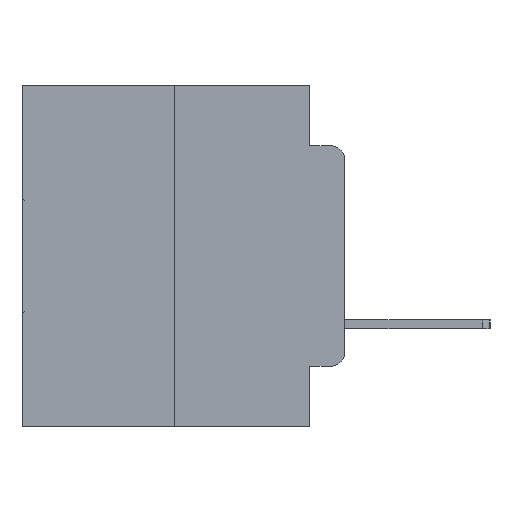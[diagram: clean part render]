
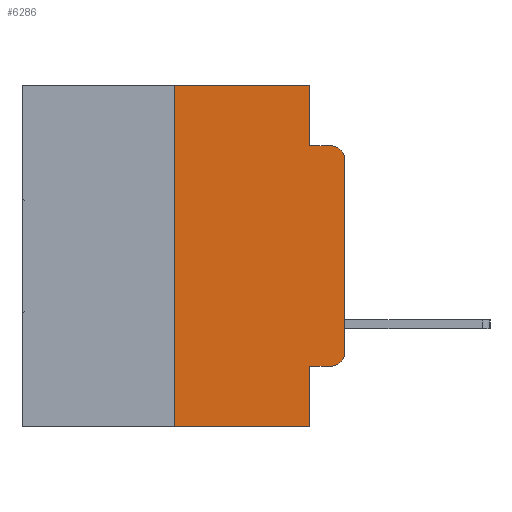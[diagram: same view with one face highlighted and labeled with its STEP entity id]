
A CAD part, left-side view. The second image highlights one B-rep face of the part: STEP entity #6286.
In plain terms, the highlighted planar face has unit normal (-1, 0, 0).
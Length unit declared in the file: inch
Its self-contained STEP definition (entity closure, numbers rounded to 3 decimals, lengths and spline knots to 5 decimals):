
#160 = CARTESIAN_POINT ( 'NONE',  ( 0., 0., -0.1085 ) ) ;
#285 = EDGE_CURVE ( 'NONE', #18609, #29116, #14256, .T. ) ;
#419 = LINE ( 'NONE', #23918, #28640 ) ;
#1270 = VERTEX_POINT ( 'NONE', #28514 ) ;
#1973 = EDGE_CURVE ( 'NONE', #26638, #18609, #24663, .T. ) ;
#2073 = LINE ( 'NONE', #5348, #7656 ) ;
#2400 = ORIENTED_EDGE ( 'NONE', *, *, #21439, .T. ) ;
#2873 = LINE ( 'NONE', #26602, #19403 ) ;
#3218 = EDGE_CURVE ( 'NONE', #14050, #19215, #4647, .T. ) ;
#3856 = CARTESIAN_POINT ( 'NONE',  ( 0., 0.02, -0.3915 ) ) ;
#4589 = AXIS2_PLACEMENT_3D ( 'NONE', #22529, #22428, #27121 ) ;
#4647 = LINE ( 'NONE', #22957, #28654 ) ;
#5004 = ORIENTED_EDGE ( 'NONE', *, *, #1973, .T. ) ;
#5060 = DIRECTION ( 'NONE',  ( 0., -1., 0. ) ) ;
#5348 = CARTESIAN_POINT ( 'NONE',  ( 0., 0.051, -0.4115 ) ) ;
#5400 = CARTESIAN_POINT ( 'NONE',  ( 0., 0., 0. ) ) ;
#5578 = VECTOR ( 'NONE', #5060, 39.37008 ) ;
#6203 = DIRECTION ( 'NONE',  ( 0., 0., -1. ) ) ;
#6286 = ADVANCED_FACE ( 'NONE', ( #17348 ), #24834, .F. ) ;
#6329 = VERTEX_POINT ( 'NONE', #27222 ) ;
#7656 = VECTOR ( 'NONE', #26346, 39.37008 ) ;
#7874 = VERTEX_POINT ( 'NONE', #24130 ) ;
#8524 = DIRECTION ( 'NONE',  ( 0., 0., -1. ) ) ;
#8939 = CARTESIAN_POINT ( 'NONE',  ( 0., 0.25, 0. ) ) ;
#8965 = EDGE_CURVE ( 'NONE', #14423, #1270, #2073, .T. ) ;
#9714 = CARTESIAN_POINT ( 'NONE',  ( 0., 0.051, 0. ) ) ;
#9726 = CARTESIAN_POINT ( 'NONE',  ( 0., 0.051, -0.0885 ) ) ;
#11994 = VERTEX_POINT ( 'NONE', #24104 ) ;
#12165 = EDGE_CURVE ( 'NONE', #14423, #11994, #23568, .T. ) ;
#12405 = CARTESIAN_POINT ( 'NONE',  ( 0., 0., -0.3915 ) ) ;
#13073 = VECTOR ( 'NONE', #24089, 39.37008 ) ;
#13245 = CARTESIAN_POINT ( 'NONE',  ( 0., 0.02, -0.1085 ) ) ;
#13515 = ORIENTED_EDGE ( 'NONE', *, *, #19920, .F. ) ;
#13523 = AXIS2_PLACEMENT_3D ( 'NONE', #3856, #20240, #6203 ) ;
#14050 = VERTEX_POINT ( 'NONE', #8939 ) ;
#14256 = CIRCLE ( 'NONE', #28641, 0.02 ) ;
#14423 = VERTEX_POINT ( 'NONE', #19727 ) ;
#14699 = DIRECTION ( 'NONE',  ( 0., 0., 1. ) ) ;
#15256 = EDGE_CURVE ( 'NONE', #7874, #14050, #419, .T. ) ;
#15309 = EDGE_LOOP ( 'NONE', ( #5004, #29695, #18971, #13515, #20412, #26522, #2400, #21862, #27959, #17120 ) ) ;
#15576 = DIRECTION ( 'NONE',  ( 0., 0., -1. ) ) ;
#16053 = DIRECTION ( 'NONE',  ( 0., -1., 0. ) ) ;
#16829 = CARTESIAN_POINT ( 'NONE',  ( 0., 0.473, -0.5 ) ) ;
#17120 = ORIENTED_EDGE ( 'NONE', *, *, #29683, .T. ) ;
#17348 = FACE_OUTER_BOUND ( 'NONE', #15309, .T. ) ;
#17412 = DIRECTION ( 'NONE',  ( 0., 0., -1. ) ) ;
#18609 = VERTEX_POINT ( 'NONE', #160 ) ;
#18971 = ORIENTED_EDGE ( 'NONE', *, *, #26090, .F. ) ;
#19198 = DIRECTION ( 'NONE',  ( 0., -1., 0. ) ) ;
#19215 = VERTEX_POINT ( 'NONE', #9714 ) ;
#19403 = VECTOR ( 'NONE', #17412, 39.37008 ) ;
#19727 = CARTESIAN_POINT ( 'NONE',  ( 0., 0.051, -0.4115 ) ) ;
#19822 = CIRCLE ( 'NONE', #13523, 0.02 ) ;
#19920 = EDGE_CURVE ( 'NONE', #19215, #6329, #2873, .T. ) ;
#20068 = CARTESIAN_POINT ( 'NONE',  ( 0., 0.02, -0.0885 ) ) ;
#20163 = CARTESIAN_POINT ( 'NONE',  ( 0., 0.051, 0. ) ) ;
#20240 = DIRECTION ( 'NONE',  ( -1., 0., 0. ) ) ;
#20412 = ORIENTED_EDGE ( 'NONE', *, *, #3218, .F. ) ;
#21439 = EDGE_CURVE ( 'NONE', #7874, #11994, #23809, .T. ) ;
#21862 = ORIENTED_EDGE ( 'NONE', *, *, #12165, .F. ) ;
#22428 = DIRECTION ( 'NONE',  ( 1., 0., 0. ) ) ;
#22529 = CARTESIAN_POINT ( 'NONE',  ( 0., 0.473, 0. ) ) ;
#22957 = CARTESIAN_POINT ( 'NONE',  ( 0., 0.473, 0. ) ) ;
#23568 = LINE ( 'NONE', #20163, #29610 ) ;
#23809 = LINE ( 'NONE', #16829, #28443 ) ;
#23918 = CARTESIAN_POINT ( 'NONE',  ( 0., 0.25, 0. ) ) ;
#24089 = DIRECTION ( 'NONE',  ( 0., 0., 1. ) ) ;
#24104 = CARTESIAN_POINT ( 'NONE',  ( 0., 0.051, -0.5 ) ) ;
#24130 = CARTESIAN_POINT ( 'NONE',  ( 0., 0.25, -0.5 ) ) ;
#24663 = LINE ( 'NONE', #5400, #13073 ) ;
#24834 = PLANE ( 'NONE',  #4589 ) ;
#26090 = EDGE_CURVE ( 'NONE', #6329, #29116, #30243, .T. ) ;
#26346 = DIRECTION ( 'NONE',  ( 0., -1., 0. ) ) ;
#26522 = ORIENTED_EDGE ( 'NONE', *, *, #15256, .F. ) ;
#26602 = CARTESIAN_POINT ( 'NONE',  ( 0., 0.051, 0. ) ) ;
#26638 = VERTEX_POINT ( 'NONE', #12405 ) ;
#27121 = DIRECTION ( 'NONE',  ( 0., 0., -1. ) ) ;
#27222 = CARTESIAN_POINT ( 'NONE',  ( 0., 0.051, -0.0885 ) ) ;
#27959 = ORIENTED_EDGE ( 'NONE', *, *, #8965, .T. ) ;
#28443 = VECTOR ( 'NONE', #19198, 39.37008 ) ;
#28514 = CARTESIAN_POINT ( 'NONE',  ( 0., 0.02, -0.4115 ) ) ;
#28640 = VECTOR ( 'NONE', #14699, 39.37008 ) ;
#28641 = AXIS2_PLACEMENT_3D ( 'NONE', #13245, #29331, #15576 ) ;
#28654 = VECTOR ( 'NONE', #16053, 39.37008 ) ;
#29116 = VERTEX_POINT ( 'NONE', #20068 ) ;
#29331 = DIRECTION ( 'NONE',  ( -1., 0., 0. ) ) ;
#29610 = VECTOR ( 'NONE', #8524, 39.37008 ) ;
#29683 = EDGE_CURVE ( 'NONE', #1270, #26638, #19822, .T. ) ;
#29695 = ORIENTED_EDGE ( 'NONE', *, *, #285, .T. ) ;
#30243 = LINE ( 'NONE', #9726, #5578 ) ;
